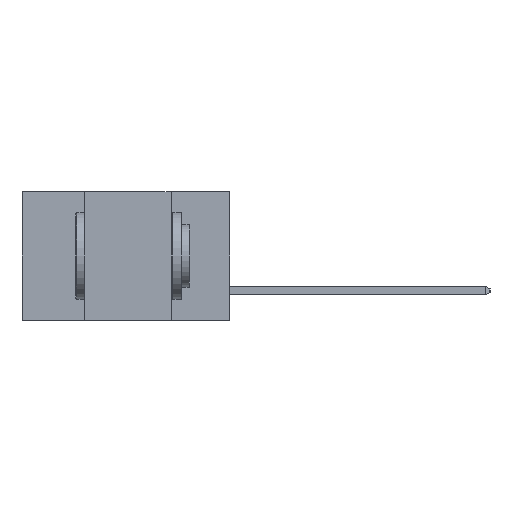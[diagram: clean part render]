
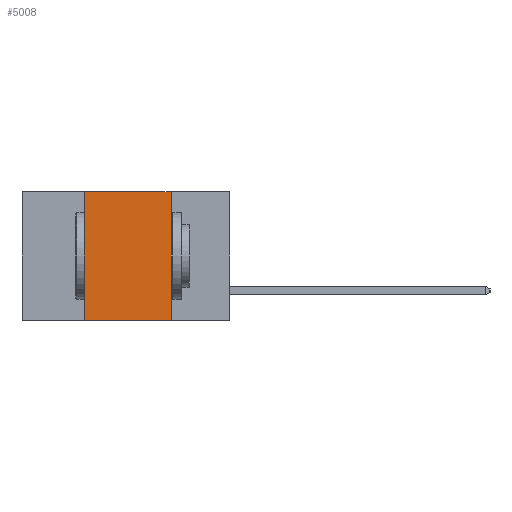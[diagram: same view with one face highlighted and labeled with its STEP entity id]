
A CAD part, left-side view. The second image highlights one B-rep face of the part: STEP entity #5008.
In plain terms, the highlighted planar face has unit normal (-1, 0, 0).
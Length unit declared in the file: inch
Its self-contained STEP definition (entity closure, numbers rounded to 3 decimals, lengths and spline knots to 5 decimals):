
#1299 = CARTESIAN_POINT ( 'NONE',  ( 0., 0.6, 0. ) ) ;
#1494 = CARTESIAN_POINT ( 'NONE',  ( 0., 0.42, -0.37 ) ) ;
#3520 = LINE ( 'NONE', #6967, #21180 ) ;
#4111 = LINE ( 'NONE', #1299, #17151 ) ;
#4323 = ORIENTED_EDGE ( 'NONE', *, *, #4591, .F. ) ;
#4591 = EDGE_CURVE ( 'NONE', #20347, #10405, #3520, .T. ) ;
#4643 = DIRECTION ( 'NONE',  ( 0., -1., 0. ) ) ;
#5008 = ADVANCED_FACE ( 'NONE', ( #21156 ), #15093, .F. ) ;
#5216 = LINE ( 'NONE', #14818, #7331 ) ;
#5825 = VECTOR ( 'NONE', #20595, 39.37008 ) ;
#5919 = CARTESIAN_POINT ( 'NONE',  ( 0., 0.17, 0. ) ) ;
#6348 = ORIENTED_EDGE ( 'NONE', *, *, #14188, .F. ) ;
#6967 = CARTESIAN_POINT ( 'NONE',  ( 0., 0.17, 0. ) ) ;
#7331 = VECTOR ( 'NONE', #4643, 39.37008 ) ;
#8039 = DIRECTION ( 'NONE',  ( 0., -1., 0. ) ) ;
#8863 = CARTESIAN_POINT ( 'NONE',  ( 0., 0.17, -0.37 ) ) ;
#9129 = VERTEX_POINT ( 'NONE', #1494 ) ;
#9811 = CARTESIAN_POINT ( 'NONE',  ( 0., 0.42, 0. ) ) ;
#10026 = ORIENTED_EDGE ( 'NONE', *, *, #14117, .T. ) ;
#10326 = LINE ( 'NONE', #20665, #5825 ) ;
#10405 = VERTEX_POINT ( 'NONE', #8863 ) ;
#10779 = VERTEX_POINT ( 'NONE', #9811 ) ;
#11438 = AXIS2_PLACEMENT_3D ( 'NONE', #11906, #11840, #11820 ) ;
#11820 = DIRECTION ( 'NONE',  ( 0., 0., -1. ) ) ;
#11840 = DIRECTION ( 'NONE',  ( 1., 0., 0. ) ) ;
#11906 = CARTESIAN_POINT ( 'NONE',  ( 0., 0.6, 0. ) ) ;
#14117 = EDGE_CURVE ( 'NONE', #9129, #10405, #5216, .T. ) ;
#14188 = EDGE_CURVE ( 'NONE', #10779, #20347, #4111, .T. ) ;
#14818 = CARTESIAN_POINT ( 'NONE',  ( 0., 0.6, -0.37 ) ) ;
#15093 = PLANE ( 'NONE',  #11438 ) ;
#16071 = ORIENTED_EDGE ( 'NONE', *, *, #17553, .F. ) ;
#17151 = VECTOR ( 'NONE', #8039, 39.37008 ) ;
#17553 = EDGE_CURVE ( 'NONE', #9129, #10779, #10326, .T. ) ;
#17938 = EDGE_LOOP ( 'NONE', ( #4323, #6348, #16071, #10026 ) ) ;
#20347 = VERTEX_POINT ( 'NONE', #5919 ) ;
#20595 = DIRECTION ( 'NONE',  ( 0., 0., 1. ) ) ;
#20665 = CARTESIAN_POINT ( 'NONE',  ( 0., 0.42, 0. ) ) ;
#21156 = FACE_OUTER_BOUND ( 'NONE', #17938, .T. ) ;
#21180 = VECTOR ( 'NONE', #21602, 39.37008 ) ;
#21602 = DIRECTION ( 'NONE',  ( 0., 0., -1. ) ) ;
